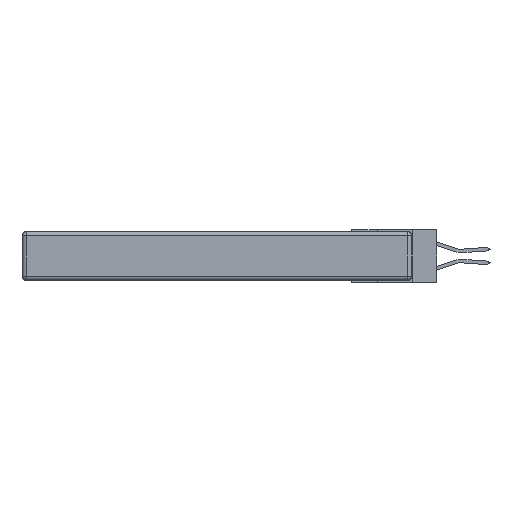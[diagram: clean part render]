
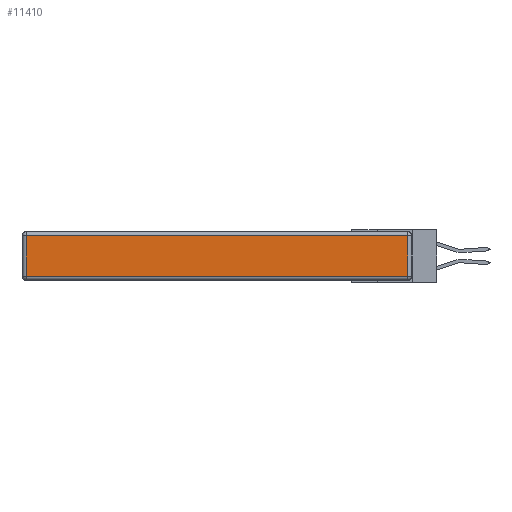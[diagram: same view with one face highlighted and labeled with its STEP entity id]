
A CAD part, left-side view. The second image highlights one B-rep face of the part: STEP entity #11410.
In plain terms, the highlighted planar face has unit normal (-1, 0, 0).
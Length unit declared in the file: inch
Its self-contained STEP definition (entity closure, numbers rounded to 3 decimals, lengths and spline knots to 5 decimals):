
#97 = DIRECTION ( 'NONE',  ( 0., 0., 1. ) ) ;
#541 = DIRECTION ( 'NONE',  ( 0., 0., -1. ) ) ;
#703 = VERTEX_POINT ( 'NONE', #5903 ) ;
#1107 = EDGE_CURVE ( 'NONE', #26656, #703, #19321, .T. ) ;
#2066 = LINE ( 'NONE', #11296, #24646 ) ;
#2478 = CARTESIAN_POINT ( 'NONE',  ( 0., 2.72, -0.313 ) ) ;
#3450 = DIRECTION ( 'NONE',  ( 0., 1., 0. ) ) ;
#5005 = ORIENTED_EDGE ( 'NONE', *, *, #19021, .T. ) ;
#5141 = EDGE_CURVE ( 'NONE', #703, #9916, #11193, .T. ) ;
#5409 = VECTOR ( 'NONE', #23137, 39.37008 ) ;
#5883 = CARTESIAN_POINT ( 'NONE',  ( 0., 2.75, -0.03 ) ) ;
#5903 = CARTESIAN_POINT ( 'NONE',  ( 0., 2.72, -0.03 ) ) ;
#8607 = VECTOR ( 'NONE', #3450, 39.37008 ) ;
#9660 = EDGE_CURVE ( 'NONE', #24946, #26656, #11158, .T. ) ;
#9916 = VERTEX_POINT ( 'NONE', #2478 ) ;
#10934 = PLANE ( 'NONE',  #19680 ) ;
#11158 = LINE ( 'NONE', #14634, #5409 ) ;
#11193 = LINE ( 'NONE', #27665, #25284 ) ;
#11296 = CARTESIAN_POINT ( 'NONE',  ( 0., 0., -0.313 ) ) ;
#11410 = ADVANCED_FACE ( 'NONE', ( #24167 ), #10934, .T. ) ;
#11918 = ORIENTED_EDGE ( 'NONE', *, *, #1107, .T. ) ;
#14634 = CARTESIAN_POINT ( 'NONE',  ( 0., 0.03, -0.343 ) ) ;
#14980 = DIRECTION ( 'NONE',  ( -1., 0., 0. ) ) ;
#19021 = EDGE_CURVE ( 'NONE', #9916, #24946, #2066, .T. ) ;
#19321 = LINE ( 'NONE', #5883, #8607 ) ;
#19680 = AXIS2_PLACEMENT_3D ( 'NONE', #23971, #14980, #97 ) ;
#20885 = ORIENTED_EDGE ( 'NONE', *, *, #5141, .T. ) ;
#21007 = CARTESIAN_POINT ( 'NONE',  ( 0., 0.03, -0.313 ) ) ;
#22926 = ORIENTED_EDGE ( 'NONE', *, *, #9660, .T. ) ;
#23137 = DIRECTION ( 'NONE',  ( 0., 0., 1. ) ) ;
#23388 = CARTESIAN_POINT ( 'NONE',  ( 0., 0.03, -0.03 ) ) ;
#23971 = CARTESIAN_POINT ( 'NONE',  ( 0., 0., -0.343 ) ) ;
#24167 = FACE_OUTER_BOUND ( 'NONE', #24478, .T. ) ;
#24478 = EDGE_LOOP ( 'NONE', ( #5005, #22926, #11918, #20885 ) ) ;
#24646 = VECTOR ( 'NONE', #26291, 39.37008 ) ;
#24946 = VERTEX_POINT ( 'NONE', #21007 ) ;
#25284 = VECTOR ( 'NONE', #541, 39.37008 ) ;
#26291 = DIRECTION ( 'NONE',  ( 0., -1., 0. ) ) ;
#26656 = VERTEX_POINT ( 'NONE', #23388 ) ;
#27665 = CARTESIAN_POINT ( 'NONE',  ( 0., 2.72, -0.343 ) ) ;
